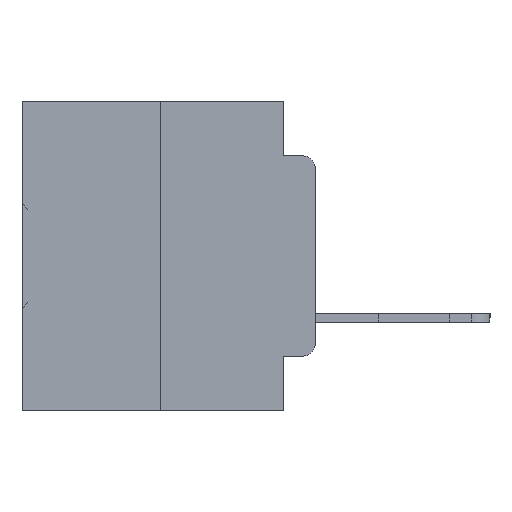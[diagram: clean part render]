
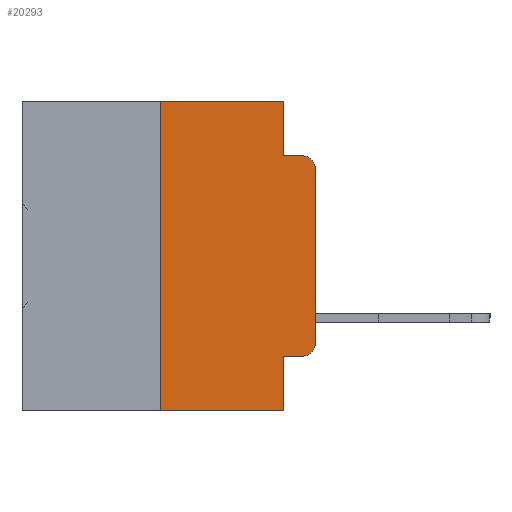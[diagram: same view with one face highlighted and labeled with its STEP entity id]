
A CAD part, left-side view. The second image highlights one B-rep face of the part: STEP entity #20293.
In plain terms, the highlighted planar face has unit normal (-1, 0, 0).
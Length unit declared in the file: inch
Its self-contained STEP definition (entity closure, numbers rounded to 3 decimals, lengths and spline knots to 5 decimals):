
#37 = VECTOR ( 'NONE', #3590, 39.37008 ) ;
#171 = VECTOR ( 'NONE', #7668, 39.37008 ) ;
#542 = CARTESIAN_POINT ( 'NONE',  ( 0., 0.051, 0. ) ) ;
#593 = VECTOR ( 'NONE', #26355, 39.37008 ) ;
#1292 = DIRECTION ( 'NONE',  ( 0., 0., -1. ) ) ;
#1322 = ORIENTED_EDGE ( 'NONE', *, *, #17481, .F. ) ;
#1882 = AXIS2_PLACEMENT_3D ( 'NONE', #32879, #17345, #1292 ) ;
#2912 = VECTOR ( 'NONE', #13393, 39.37008 ) ;
#3590 = DIRECTION ( 'NONE',  ( 0., 0., -1. ) ) ;
#3652 = CARTESIAN_POINT ( 'NONE',  ( 0., 0.051, -0.4115 ) ) ;
#3661 = CARTESIAN_POINT ( 'NONE',  ( 0., 0.25, 0. ) ) ;
#3893 = CARTESIAN_POINT ( 'NONE',  ( 0., 0.02, -0.4115 ) ) ;
#4491 = VERTEX_POINT ( 'NONE', #3661 ) ;
#4632 = VECTOR ( 'NONE', #32974, 39.37008 ) ;
#4633 = DIRECTION ( 'NONE',  ( 1., 0., 0. ) ) ;
#4835 = CARTESIAN_POINT ( 'NONE',  ( 0., 0.02, -0.1085 ) ) ;
#4980 = EDGE_CURVE ( 'NONE', #11728, #18832, #26821, .T. ) ;
#5227 = CARTESIAN_POINT ( 'NONE',  ( 0., 0.051, 0. ) ) ;
#5604 = ORIENTED_EDGE ( 'NONE', *, *, #6599, .T. ) ;
#5640 = LINE ( 'NONE', #19515, #37 ) ;
#6426 = DIRECTION ( 'NONE',  ( 0., -1., 0. ) ) ;
#6599 = EDGE_CURVE ( 'NONE', #6873, #16217, #9876, .T. ) ;
#6873 = VERTEX_POINT ( 'NONE', #11026 ) ;
#7586 = DIRECTION ( 'NONE',  ( 0., 0., -1. ) ) ;
#7668 = DIRECTION ( 'NONE',  ( 0., 0., 1. ) ) ;
#8051 = VERTEX_POINT ( 'NONE', #29481 ) ;
#8469 = LINE ( 'NONE', #21262, #2912 ) ;
#8524 = EDGE_CURVE ( 'NONE', #4491, #32555, #8469, .T. ) ;
#8916 = VECTOR ( 'NONE', #6426, 39.37008 ) ;
#9876 = LINE ( 'NONE', #19999, #22163 ) ;
#10314 = CARTESIAN_POINT ( 'NONE',  ( 0., 0., -0.3915 ) ) ;
#10394 = EDGE_CURVE ( 'NONE', #18832, #8051, #21290, .T. ) ;
#11026 = CARTESIAN_POINT ( 'NONE',  ( 0., 0.25, -0.5 ) ) ;
#11728 = VERTEX_POINT ( 'NONE', #10314 ) ;
#11805 = LINE ( 'NONE', #14711, #4632 ) ;
#12214 = EDGE_CURVE ( 'NONE', #31059, #8051, #19994, .T. ) ;
#13050 = VECTOR ( 'NONE', #25790, 39.37008 ) ;
#13286 = AXIS2_PLACEMENT_3D ( 'NONE', #4835, #23327, #7586 ) ;
#13393 = DIRECTION ( 'NONE',  ( 0., -1., 0. ) ) ;
#13994 = EDGE_CURVE ( 'NONE', #32555, #31059, #5640, .T. ) ;
#14711 = CARTESIAN_POINT ( 'NONE',  ( 0., 0.25, 0. ) ) ;
#15339 = CARTESIAN_POINT ( 'NONE',  ( 0., 0.473, 0. ) ) ;
#15782 = EDGE_CURVE ( 'NONE', #6873, #4491, #11805, .T. ) ;
#16217 = VERTEX_POINT ( 'NONE', #32367 ) ;
#16241 = ORIENTED_EDGE ( 'NONE', *, *, #12214, .F. ) ;
#17345 = DIRECTION ( 'NONE',  ( -1., 0., 0. ) ) ;
#17481 = EDGE_CURVE ( 'NONE', #22991, #16217, #29582, .T. ) ;
#17893 = PLANE ( 'NONE',  #29070 ) ;
#18806 = ORIENTED_EDGE ( 'NONE', *, *, #19215, .T. ) ;
#18832 = VERTEX_POINT ( 'NONE', #23125 ) ;
#19215 = EDGE_CURVE ( 'NONE', #22991, #19297, #29774, .T. ) ;
#19297 = VERTEX_POINT ( 'NONE', #3893 ) ;
#19515 = CARTESIAN_POINT ( 'NONE',  ( 0., 0.051, 0. ) ) ;
#19994 = LINE ( 'NONE', #33481, #13050 ) ;
#19999 = CARTESIAN_POINT ( 'NONE',  ( 0., 0.473, -0.5 ) ) ;
#20000 = FACE_OUTER_BOUND ( 'NONE', #27995, .T. ) ;
#20293 = ADVANCED_FACE ( 'NONE', ( #20000 ), #17893, .F. ) ;
#20875 = ORIENTED_EDGE ( 'NONE', *, *, #15782, .F. ) ;
#21262 = CARTESIAN_POINT ( 'NONE',  ( 0., 0.473, 0. ) ) ;
#21290 = CIRCLE ( 'NONE', #13286, 0.02 ) ;
#22163 = VECTOR ( 'NONE', #25164, 39.37008 ) ;
#22698 = EDGE_CURVE ( 'NONE', #19297, #11728, #27457, .T. ) ;
#22991 = VERTEX_POINT ( 'NONE', #31024 ) ;
#23125 = CARTESIAN_POINT ( 'NONE',  ( 0., 0., -0.1085 ) ) ;
#23128 = DIRECTION ( 'NONE',  ( 0., 0., -1. ) ) ;
#23327 = DIRECTION ( 'NONE',  ( -1., 0., 0. ) ) ;
#23407 = CARTESIAN_POINT ( 'NONE',  ( 0., 0., 0. ) ) ;
#25164 = DIRECTION ( 'NONE',  ( 0., -1., 0. ) ) ;
#25790 = DIRECTION ( 'NONE',  ( 0., -1., 0. ) ) ;
#26355 = DIRECTION ( 'NONE',  ( 0., 0., -1. ) ) ;
#26821 = LINE ( 'NONE', #23407, #171 ) ;
#27457 = CIRCLE ( 'NONE', #1882, 0.02 ) ;
#27995 = EDGE_LOOP ( 'NONE', ( #31527, #32750, #16241, #33163, #30679, #20875, #5604, #1322, #18806, #30246 ) ) ;
#28691 = CARTESIAN_POINT ( 'NONE',  ( 0., 0.051, -0.0885 ) ) ;
#29070 = AXIS2_PLACEMENT_3D ( 'NONE', #15339, #4633, #23128 ) ;
#29481 = CARTESIAN_POINT ( 'NONE',  ( 0., 0.02, -0.0885 ) ) ;
#29582 = LINE ( 'NONE', #5227, #593 ) ;
#29774 = LINE ( 'NONE', #3652, #8916 ) ;
#30246 = ORIENTED_EDGE ( 'NONE', *, *, #22698, .T. ) ;
#30679 = ORIENTED_EDGE ( 'NONE', *, *, #8524, .F. ) ;
#31024 = CARTESIAN_POINT ( 'NONE',  ( 0., 0.051, -0.4115 ) ) ;
#31059 = VERTEX_POINT ( 'NONE', #28691 ) ;
#31527 = ORIENTED_EDGE ( 'NONE', *, *, #4980, .T. ) ;
#32367 = CARTESIAN_POINT ( 'NONE',  ( 0., 0.051, -0.5 ) ) ;
#32555 = VERTEX_POINT ( 'NONE', #542 ) ;
#32750 = ORIENTED_EDGE ( 'NONE', *, *, #10394, .T. ) ;
#32879 = CARTESIAN_POINT ( 'NONE',  ( 0., 0.02, -0.3915 ) ) ;
#32974 = DIRECTION ( 'NONE',  ( 0., 0., 1. ) ) ;
#33163 = ORIENTED_EDGE ( 'NONE', *, *, #13994, .F. ) ;
#33481 = CARTESIAN_POINT ( 'NONE',  ( 0., 0.051, -0.0885 ) ) ;
